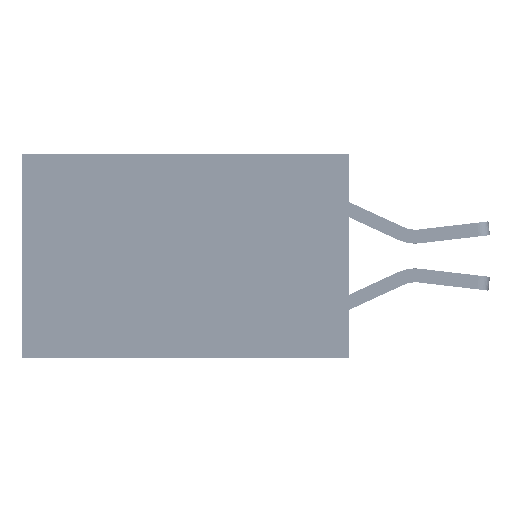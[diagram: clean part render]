
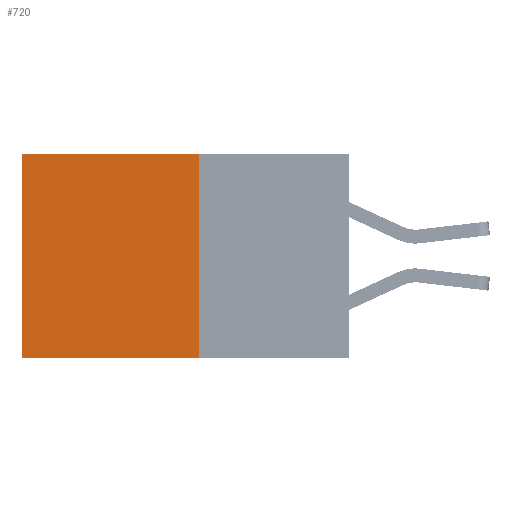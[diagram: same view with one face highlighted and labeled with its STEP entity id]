
A CAD part, left-side view. The second image highlights one B-rep face of the part: STEP entity #720.
In plain terms, the highlighted planar face has unit normal (-1, 0, 0).
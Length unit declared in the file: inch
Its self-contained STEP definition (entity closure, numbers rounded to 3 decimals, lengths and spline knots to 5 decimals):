
#52 = CARTESIAN_POINT ( 'NONE',  ( 0.277, 0.27, 0. ) ) ;
#720 = ADVANCED_FACE ( 'NONE', ( #838 ), #29538, .F. ) ;
#790 = EDGE_CURVE ( 'NONE', #3030, #31035, #13232, .T. ) ;
#838 = FACE_OUTER_BOUND ( 'NONE', #4296, .T. ) ;
#2629 = ORIENTED_EDGE ( 'NONE', *, *, #790, .F. ) ;
#3030 = VERTEX_POINT ( 'NONE', #3871 ) ;
#3871 = CARTESIAN_POINT ( 'NONE',  ( 0.277, 0.27, 0. ) ) ;
#4296 = EDGE_LOOP ( 'NONE', ( #24735, #32248, #2629, #14194 ) ) ;
#5195 = LINE ( 'NONE', #52, #18446 ) ;
#6119 = EDGE_CURVE ( 'NONE', #3030, #15764, #5195, .T. ) ;
#7425 = CARTESIAN_POINT ( 'NONE',  ( 0.277, 0.27, -0.37 ) ) ;
#7631 = LINE ( 'NONE', #7425, #20898 ) ;
#11200 = DIRECTION ( 'NONE',  ( 1., 0., 0. ) ) ;
#11550 = DIRECTION ( 'NONE',  ( 0., 0., -1. ) ) ;
#11700 = VERTEX_POINT ( 'NONE', #26444 ) ;
#11972 = VECTOR ( 'NONE', #11550, 39.37008 ) ;
#12271 = EDGE_CURVE ( 'NONE', #31035, #11700, #7631, .T. ) ;
#13232 = LINE ( 'NONE', #20174, #26459 ) ;
#14194 = ORIENTED_EDGE ( 'NONE', *, *, #6119, .T. ) ;
#14586 = EDGE_CURVE ( 'NONE', #15764, #11700, #18188, .T. ) ;
#15764 = VERTEX_POINT ( 'NONE', #31770 ) ;
#17594 = CARTESIAN_POINT ( 'NONE',  ( 0.277, 0.27, -0.37 ) ) ;
#18081 = DIRECTION ( 'NONE',  ( 0., 1., 0. ) ) ;
#18188 = LINE ( 'NONE', #24754, #11972 ) ;
#18319 = AXIS2_PLACEMENT_3D ( 'NONE', #17594, #11200, #29833 ) ;
#18446 = VECTOR ( 'NONE', #31613, 39.37008 ) ;
#20174 = CARTESIAN_POINT ( 'NONE',  ( 0.277, 0.27, -0.37 ) ) ;
#20586 = CARTESIAN_POINT ( 'NONE',  ( 0.277, 0.27, -0.37 ) ) ;
#20898 = VECTOR ( 'NONE', #18081, 39.37008 ) ;
#24705 = DIRECTION ( 'NONE',  ( 0., 0., -1. ) ) ;
#24735 = ORIENTED_EDGE ( 'NONE', *, *, #14586, .T. ) ;
#24754 = CARTESIAN_POINT ( 'NONE',  ( 0.277, 0.59, -0.37 ) ) ;
#26444 = CARTESIAN_POINT ( 'NONE',  ( 0.277, 0.59, -0.37 ) ) ;
#26459 = VECTOR ( 'NONE', #24705, 39.37008 ) ;
#29538 = PLANE ( 'NONE',  #18319 ) ;
#29833 = DIRECTION ( 'NONE',  ( 0., 0., -1. ) ) ;
#31035 = VERTEX_POINT ( 'NONE', #20586 ) ;
#31613 = DIRECTION ( 'NONE',  ( 0., 1., 0. ) ) ;
#31770 = CARTESIAN_POINT ( 'NONE',  ( 0.277, 0.59, 0. ) ) ;
#32248 = ORIENTED_EDGE ( 'NONE', *, *, #12271, .F. ) ;
